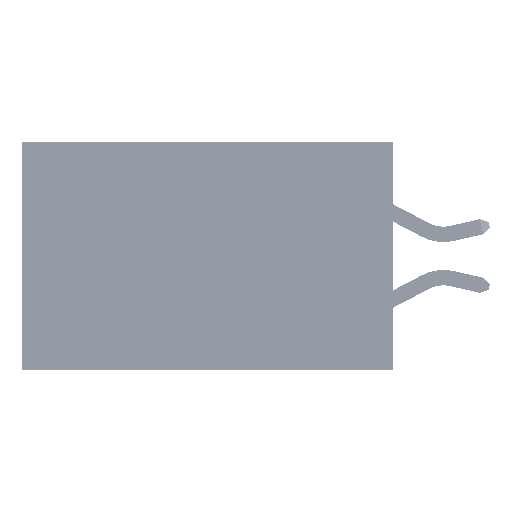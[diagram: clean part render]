
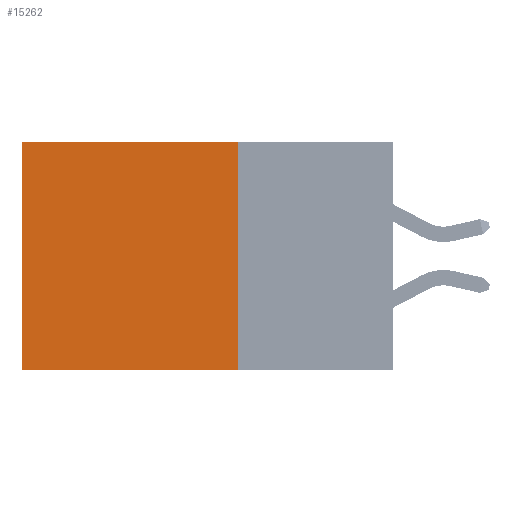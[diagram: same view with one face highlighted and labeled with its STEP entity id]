
A CAD part, left-side view. The second image highlights one B-rep face of the part: STEP entity #15262.
In plain terms, the highlighted planar face has unit normal (-1, 0, 0).
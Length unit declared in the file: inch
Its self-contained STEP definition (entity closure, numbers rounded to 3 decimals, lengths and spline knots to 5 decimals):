
#41 = LINE ( 'NONE', #9310, #9131 ) ;
#2692 = EDGE_CURVE ( 'NONE', #15149, #44160, #21583, .T. ) ;
#3946 = ORIENTED_EDGE ( 'NONE', *, *, #18603, .F. ) ;
#6013 = LINE ( 'NONE', #32413, #16805 ) ;
#8307 = ORIENTED_EDGE ( 'NONE', *, *, #44418, .F. ) ;
#9131 = VECTOR ( 'NONE', #16780, 39.37008 ) ;
#9310 = CARTESIAN_POINT ( 'NONE',  ( 0.2875, 0.25, -0.37 ) ) ;
#9423 = VERTEX_POINT ( 'NONE', #10523 ) ;
#10523 = CARTESIAN_POINT ( 'NONE',  ( 0.2875, 0.6, -0.37 ) ) ;
#12968 = EDGE_LOOP ( 'NONE', ( #18360, #3946, #8307, #31639 ) ) ;
#14033 = CARTESIAN_POINT ( 'NONE',  ( 0.2875, 0.25, 0. ) ) ;
#15149 = VERTEX_POINT ( 'NONE', #36715 ) ;
#15262 = ADVANCED_FACE ( 'NONE', ( #40951 ), #26264, .F. ) ;
#16780 = DIRECTION ( 'NONE',  ( 0., 1., 0. ) ) ;
#16805 = VECTOR ( 'NONE', #46454, 39.37008 ) ;
#18360 = ORIENTED_EDGE ( 'NONE', *, *, #40683, .T. ) ;
#18603 = EDGE_CURVE ( 'NONE', #28340, #9423, #41, .T. ) ;
#21583 = LINE ( 'NONE', #14033, #25512 ) ;
#22940 = DIRECTION ( 'NONE',  ( 0., 0., -1. ) ) ;
#25512 = VECTOR ( 'NONE', #43579, 39.37008 ) ;
#25861 = CARTESIAN_POINT ( 'NONE',  ( 0.2875, 0.6, 0. ) ) ;
#26264 = PLANE ( 'NONE',  #37793 ) ;
#28340 = VERTEX_POINT ( 'NONE', #35869 ) ;
#29169 = DIRECTION ( 'NONE',  ( 0., 0., -1. ) ) ;
#30246 = LINE ( 'NONE', #25861, #43730 ) ;
#31639 = ORIENTED_EDGE ( 'NONE', *, *, #2692, .T. ) ;
#32413 = CARTESIAN_POINT ( 'NONE',  ( 0.2875, 0.25, 0. ) ) ;
#35869 = CARTESIAN_POINT ( 'NONE',  ( 0.2875, 0.25, -0.37 ) ) ;
#36715 = CARTESIAN_POINT ( 'NONE',  ( 0.2875, 0.25, 0. ) ) ;
#37793 = AXIS2_PLACEMENT_3D ( 'NONE', #40795, #41251, #22940 ) ;
#40683 = EDGE_CURVE ( 'NONE', #44160, #9423, #30246, .T. ) ;
#40795 = CARTESIAN_POINT ( 'NONE',  ( 0.2875, 0.25, 0. ) ) ;
#40951 = FACE_OUTER_BOUND ( 'NONE', #12968, .T. ) ;
#41251 = DIRECTION ( 'NONE',  ( 1., 0., 0. ) ) ;
#43579 = DIRECTION ( 'NONE',  ( 0., 1., 0. ) ) ;
#43730 = VECTOR ( 'NONE', #29169, 39.37008 ) ;
#44160 = VERTEX_POINT ( 'NONE', #45226 ) ;
#44418 = EDGE_CURVE ( 'NONE', #15149, #28340, #6013, .T. ) ;
#45226 = CARTESIAN_POINT ( 'NONE',  ( 0.2875, 0.6, 0. ) ) ;
#46454 = DIRECTION ( 'NONE',  ( 0., 0., -1. ) ) ;
